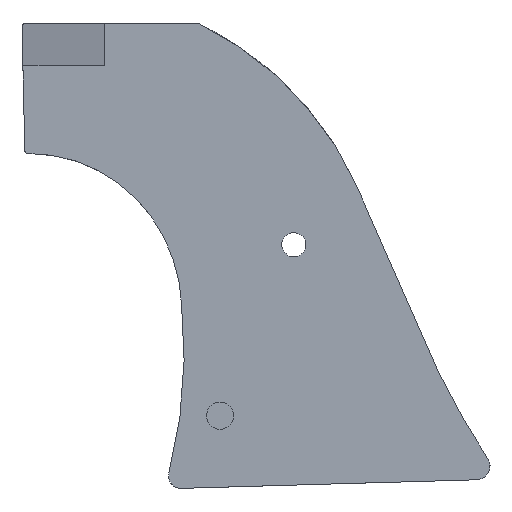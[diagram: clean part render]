
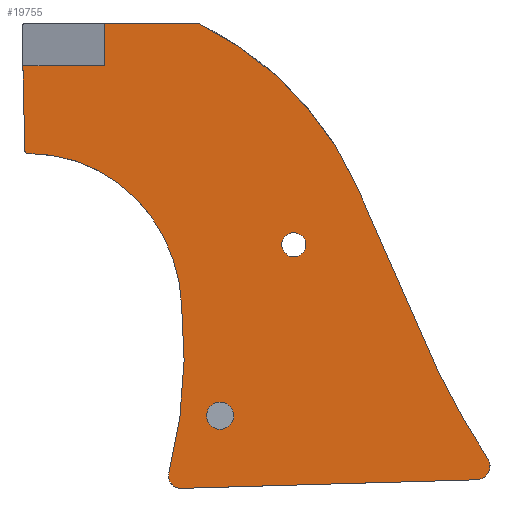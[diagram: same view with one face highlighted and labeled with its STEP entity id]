
A CAD part, left-side view. The second image highlights one B-rep face of the part: STEP entity #19755.
In plain terms, the highlighted planar face has unit normal (-1, 0, 0).
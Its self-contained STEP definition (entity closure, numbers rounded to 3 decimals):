
#3353=LINE('',#37179,#4910);
#3370=LINE('',#37532,#4927);
#3374=LINE('',#37542,#4931);
#3375=LINE('',#37545,#4932);
#3376=LINE('',#37547,#4933);
#3377=LINE('',#37550,#4934);
#3378=LINE('',#37552,#4935);
#3379=LINE('',#37553,#4936);
#4910=VECTOR('',#23205,10.);
#4927=VECTOR('',#23288,10.);
#4931=VECTOR('',#23296,10.);
#4932=VECTOR('',#23299,10.);
#4933=VECTOR('',#23300,10.);
#4934=VECTOR('',#23303,10.);
#4935=VECTOR('',#23304,10.);
#4936=VECTOR('',#23305,10.);
#5059=FACE_BOUND('',#7268,.T.);
#5060=FACE_BOUND('',#7269,.T.);
#6127=FACE_OUTER_BOUND('',#7267,.T.);
#7267=EDGE_LOOP('',(#18081,#18082,#18083,#18084,#18085,#18086,#18087,#18088,
#18089,#18090,#18091,#18092,#18093,#18094,#18095,#18096,#18097,#18098));
#7268=EDGE_LOOP('',(#18099));
#7269=EDGE_LOOP('',(#18100));
#7430=CIRCLE('',#20381,2.);
#7437=CIRCLE('',#20392,2.);
#7438=CIRCLE('',#20394,78.627);
#7446=CIRCLE('',#20413,0.5);
#7453=CIRCLE('',#20423,0.5);
#7458=CIRCLE('',#20431,25.021);
#7459=CIRCLE('',#20434,2.096);
#7460=CIRCLE('',#20435,2.353);
#7461=CIRCLE('',#20436,54.617);
#7462=CIRCLE('',#20437,27.174);
#7463=CIRCLE('',#20438,2.25);
#7464=CIRCLE('',#20439,2.);
#9326=VERTEX_POINT('',#36852);
#9327=VERTEX_POINT('',#36853);
#9338=VERTEX_POINT('',#37148);
#9339=VERTEX_POINT('',#37149);
#9340=VERTEX_POINT('',#37154);
#9343=VERTEX_POINT('',#37177);
#9358=VERTEX_POINT('',#37387);
#9359=VERTEX_POINT('',#37388);
#9371=VERTEX_POINT('',#37514);
#9372=VERTEX_POINT('',#37515);
#9374=VERTEX_POINT('',#37527);
#9375=VERTEX_POINT('',#37531);
#9378=VERTEX_POINT('',#37539);
#9379=VERTEX_POINT('',#37541);
#9380=VERTEX_POINT('',#37544);
#9381=VERTEX_POINT('',#37546);
#9382=VERTEX_POINT('',#37549);
#9383=VERTEX_POINT('',#37551);
#9384=VERTEX_POINT('',#37555);
#9385=VERTEX_POINT('',#37557);
#12232=EDGE_CURVE('',#9326,#9327,#7430,.T.);
#12250=EDGE_CURVE('',#9338,#9339,#7437,.T.);
#12253=EDGE_CURVE('',#9326,#9340,#7438,.T.);
#12260=EDGE_CURVE('',#9343,#9339,#3353,.T.);
#12283=EDGE_CURVE('',#9358,#9359,#7446,.T.);
#12300=EDGE_CURVE('',#9371,#9372,#7453,.T.);
#12308=EDGE_CURVE('',#9374,#9359,#7458,.T.);
#12309=EDGE_CURVE('',#9358,#9375,#3370,.T.);
#12313=EDGE_CURVE('',#9378,#9327,#7459,.T.);
#12314=EDGE_CURVE('',#9379,#9378,#3374,.T.);
#12315=EDGE_CURVE('',#9338,#9379,#7460,.T.);
#12316=EDGE_CURVE('',#9380,#9343,#3375,.T.);
#12317=EDGE_CURVE('',#9381,#9380,#3376,.T.);
#12318=EDGE_CURVE('',#9371,#9381,#7461,.T.);
#12319=EDGE_CURVE('',#9382,#9372,#3377,.T.);
#12320=EDGE_CURVE('',#9383,#9382,#3378,.T.);
#12321=EDGE_CURVE('',#9375,#9383,#3379,.T.);
#12322=EDGE_CURVE('',#9340,#9374,#7462,.T.);
#12323=EDGE_CURVE('',#9384,#9384,#7463,.T.);
#12324=EDGE_CURVE('',#9385,#9385,#7464,.T.);
#18081=ORIENTED_EDGE('',*,*,#12232,.T.);
#18082=ORIENTED_EDGE('',*,*,#12313,.F.);
#18083=ORIENTED_EDGE('',*,*,#12314,.F.);
#18084=ORIENTED_EDGE('',*,*,#12315,.F.);
#18085=ORIENTED_EDGE('',*,*,#12250,.T.);
#18086=ORIENTED_EDGE('',*,*,#12260,.F.);
#18087=ORIENTED_EDGE('',*,*,#12316,.F.);
#18088=ORIENTED_EDGE('',*,*,#12317,.F.);
#18089=ORIENTED_EDGE('',*,*,#12318,.F.);
#18090=ORIENTED_EDGE('',*,*,#12300,.T.);
#18091=ORIENTED_EDGE('',*,*,#12319,.F.);
#18092=ORIENTED_EDGE('',*,*,#12320,.F.);
#18093=ORIENTED_EDGE('',*,*,#12321,.F.);
#18094=ORIENTED_EDGE('',*,*,#12309,.F.);
#18095=ORIENTED_EDGE('',*,*,#12283,.T.);
#18096=ORIENTED_EDGE('',*,*,#12308,.F.);
#18097=ORIENTED_EDGE('',*,*,#12322,.F.);
#18098=ORIENTED_EDGE('',*,*,#12253,.F.);
#18099=ORIENTED_EDGE('',*,*,#12323,.F.);
#18100=ORIENTED_EDGE('',*,*,#12324,.F.);
#18679=PLANE('',#20433);
#19755=ADVANCED_FACE('',(#6127,#5059,#5060),#18679,.F.);
#20381=AXIS2_PLACEMENT_3D('',#36854,#23159,#23160);
#20392=AXIS2_PLACEMENT_3D('',#37150,#23184,#23185);
#20394=AXIS2_PLACEMENT_3D('',#37155,#23190,#23191);
#20413=AXIS2_PLACEMENT_3D('',#37389,#23239,#23240);
#20423=AXIS2_PLACEMENT_3D('',#37516,#23265,#23266);
#20431=AXIS2_PLACEMENT_3D('',#37529,#23284,#23285);
#20433=AXIS2_PLACEMENT_3D('',#37538,#23292,#23293);
#20434=AXIS2_PLACEMENT_3D('',#37540,#23294,#23295);
#20435=AXIS2_PLACEMENT_3D('',#37543,#23297,#23298);
#20436=AXIS2_PLACEMENT_3D('',#37548,#23301,#23302);
#20437=AXIS2_PLACEMENT_3D('',#37554,#23306,#23307);
#20438=AXIS2_PLACEMENT_3D('',#37556,#23308,#23309);
#20439=AXIS2_PLACEMENT_3D('',#37558,#23310,#23311);
#23159=DIRECTION('center_axis',(-1.,0.,0.));
#23160=DIRECTION('ref_axis',(0.,0.999,0.048));
#23184=DIRECTION('center_axis',(-1.,0.,0.));
#23185=DIRECTION('ref_axis',(0.,-0.961,0.276));
#23190=DIRECTION('center_axis',(-1.,0.,0.));
#23191=DIRECTION('ref_axis',(0.,-0.995,0.104));
#23205=DIRECTION('',(0.,-0.523,-0.852));
#23239=DIRECTION('center_axis',(-1.,0.,0.));
#23240=DIRECTION('ref_axis',(0.,0.698,-0.716));
#23265=DIRECTION('center_axis',(-1.,0.,0.));
#23266=DIRECTION('ref_axis',(0.,-0.223,0.975));
#23284=DIRECTION('center_axis',(-1.,0.,0.));
#23285=DIRECTION('ref_axis',(0.,0.023,1.));
#23288=DIRECTION('',(0.,0.023,1.));
#23292=DIRECTION('center_axis',(1.,0.,0.));
#23293=DIRECTION('ref_axis',(0.,1.,0.));
#23294=DIRECTION('center_axis',(1.,0.,0.));
#23295=DIRECTION('ref_axis',(0.,-0.029,-1.));
#23296=DIRECTION('',(0.,1.,-0.029));
#23297=DIRECTION('center_axis',(1.,0.,0.));
#23298=DIRECTION('ref_axis',(0.,-0.942,0.336));
#23299=DIRECTION('',(0.,-0.469,-0.883));
#23300=DIRECTION('',(0.,-0.403,-0.915));
#23301=DIRECTION('center_axis',(1.,0.,0.));
#23302=DIRECTION('ref_axis',(0.,-0.433,0.901));
#23303=DIRECTION('',(0.,-1.,0.));
#23304=DIRECTION('',(0.,0.,1.));
#23305=DIRECTION('',(0.,-1.,0.));
#23306=DIRECTION('center_axis',(-1.,0.,0.));
#23307=DIRECTION('ref_axis',(0.,-0.814,0.58));
#23308=DIRECTION('center_axis',(-1.,0.,0.));
#23309=DIRECTION('ref_axis',(0.,-1.,0.));
#23310=DIRECTION('center_axis',(-1.,0.,0.));
#23311=DIRECTION('ref_axis',(0.,-1.,0.));
#36852=CARTESIAN_POINT('',(3.808,-12.899,-314.573));
#36853=CARTESIAN_POINT('',(3.808,-12.859,-315.392));
#36854=CARTESIAN_POINT('Origin',(3.808,-14.834,-315.077));
#37148=CARTESIAN_POINT('',(3.808,-66.103,-313.365));
#37149=CARTESIAN_POINT('',(3.808,-65.807,-312.336));
#37150=CARTESIAN_POINT('Origin',(3.808,-64.103,-313.381));
#37154=CARTESIAN_POINT('',(3.808,-15.002,-286.617));
#37155=CARTESIAN_POINT('Origin',(3.808,63.199,-294.792));
#37177=CARTESIAN_POINT('',(3.808,-61.669,-305.59));
#37179=CARTESIAN_POINT('',(3.808,-61.669,-305.59));
#37387=CARTESIAN_POINT('',(3.808,10.978,-261.177));
#37388=CARTESIAN_POINT('',(3.808,10.477,-261.666));
#37389=CARTESIAN_POINT('Origin',(3.808,10.478,-261.166));
#37514=CARTESIAN_POINT('',(3.808,-17.907,-240.205));
#37515=CARTESIAN_POINT('',(3.808,-17.689,-240.155));
#37516=CARTESIAN_POINT('Origin',(3.808,-17.689,-240.655));
#37527=CARTESIAN_POINT('',(3.808,-9.99,-272.167));
#37529=CARTESIAN_POINT('Origin',(3.808,10.387,-286.686));
#37531=CARTESIAN_POINT('',(3.808,11.295,-247.158));
#37532=CARTESIAN_POINT('',(3.808,11.454,-240.155));
#37538=CARTESIAN_POINT('Origin',(3.808,-27.324,-278.656));
#37539=CARTESIAN_POINT('',(3.808,-14.99,-317.157));
#37540=CARTESIAN_POINT('Origin',(3.808,-14.929,-315.061));
#37541=CARTESIAN_POINT('',(3.808,-63.818,-315.737));
#37542=CARTESIAN_POINT('',(3.808,-63.818,-315.737));
#37543=CARTESIAN_POINT('Origin',(3.808,-63.749,-313.384));
#37544=CARTESIAN_POINT('',(3.808,-57.611,-297.958));
#37545=CARTESIAN_POINT('',(3.808,-57.611,-297.958));
#37546=CARTESIAN_POINT('',(3.808,-44.15,-267.383));
#37547=CARTESIAN_POINT('',(3.808,-44.15,-267.383));
#37548=CARTESIAN_POINT('Origin',(3.808,5.837,-289.391));
#37549=CARTESIAN_POINT('',(3.808,-2.225,-240.155));
#37550=CARTESIAN_POINT('',(3.808,11.454,-240.155));
#37551=CARTESIAN_POINT('',(3.808,-2.225,-247.158));
#37552=CARTESIAN_POINT('',(3.808,-2.225,-262.907));
#37553=CARTESIAN_POINT('',(3.808,-8.015,-247.158));
#37554=CARTESIAN_POINT('Origin',(3.808,12.141,-287.936));
#37555=CARTESIAN_POINT('',(3.808,-19.129,-305.119));
#37556=CARTESIAN_POINT('Origin',(3.808,-21.379,-305.119));
#37557=CARTESIAN_POINT('',(3.808,-31.595,-276.79));
#37558=CARTESIAN_POINT('Origin',(3.808,-33.595,-276.79));
